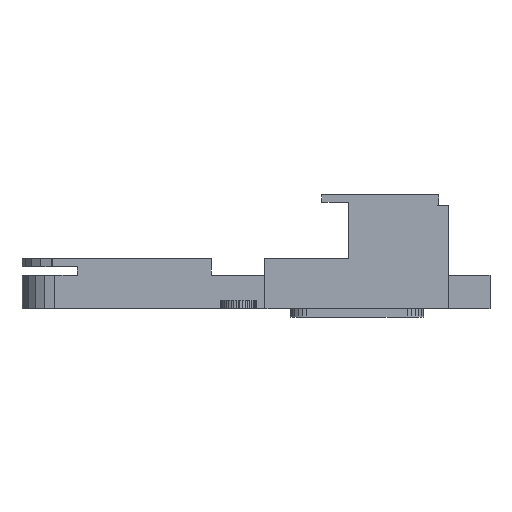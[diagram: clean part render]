
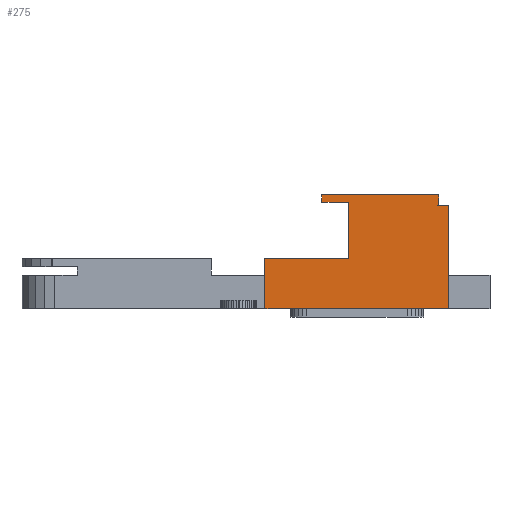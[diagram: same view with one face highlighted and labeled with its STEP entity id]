
A CAD part, front view. The second image highlights one B-rep face of the part: STEP entity #275.
In plain terms, the highlighted planar face has unit normal (0, -1, 0).
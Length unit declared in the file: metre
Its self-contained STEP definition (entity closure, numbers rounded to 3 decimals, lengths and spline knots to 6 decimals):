
#275=ADVANCED_FACE('0:2175',(#930),#931,.T.);
#930=FACE_OUTER_BOUND('',#1837,.T.);
#931=PLANE('',#1838);
#1837=EDGE_LOOP('',(#4191,#4192,#4193,#4194,#4195,#4196,#4197,#4198,#4199,#4200));
#1838=AXIS2_PLACEMENT_3D('',#4201,#4202,#4203);
#4191=ORIENTED_EDGE('',*,*,#6850,.F.);
#4192=ORIENTED_EDGE('',*,*,#6811,.F.);
#4193=ORIENTED_EDGE('',*,*,#6958,.T.);
#4194=ORIENTED_EDGE('',*,*,#6971,.T.);
#4195=ORIENTED_EDGE('',*,*,#6972,.F.);
#4196=ORIENTED_EDGE('',*,*,#6973,.T.);
#4197=ORIENTED_EDGE('',*,*,#6974,.T.);
#4198=ORIENTED_EDGE('',*,*,#6975,.T.);
#4199=ORIENTED_EDGE('',*,*,#6976,.T.);
#4200=ORIENTED_EDGE('',*,*,#6977,.F.);
#4201=CARTESIAN_POINT('',(0.019235,0.127931,0.01905));
#4202=DIRECTION('',(0.0,-1.,0.));
#4203=DIRECTION('',(0.0,0.,-1.));
#6811=EDGE_CURVE('0:2646',#8501,#8503,#8504,.T.);
#6850=EDGE_CURVE('0:2763',#8503,#8570,#8571,.T.);
#6958=EDGE_CURVE('0:3087',#8501,#8783,#8785,.T.);
#6971=EDGE_CURVE('0:3126',#8783,#8810,#8811,.T.);
#6972=EDGE_CURVE('0:3129',#8812,#8810,#8813,.T.);
#6973=EDGE_CURVE('0:3132',#8812,#8814,#8815,.T.);
#6974=EDGE_CURVE('0:3135',#8814,#8816,#8817,.T.);
#6975=EDGE_CURVE('0:3138',#8816,#8818,#8819,.T.);
#6976=EDGE_CURVE('0:3141',#8818,#8820,#8821,.T.);
#6977=EDGE_CURVE('0:3144',#8570,#8820,#8822,.T.);
#8501=VERTEX_POINT('',#11246);
#8503=VERTEX_POINT('',#11249);
#8504=LINE('',#11250,#11251);
#8570=VERTEX_POINT('',#11355);
#8571=LINE('',#11356,#11357);
#8783=VERTEX_POINT('',#11675);
#8785=LINE('',#11678,#11679);
#8810=VERTEX_POINT('',#11716);
#8811=LINE('',#11717,#11718);
#8812=VERTEX_POINT('',#11719);
#8813=LINE('',#11720,#11721);
#8814=VERTEX_POINT('',#11722);
#8815=LINE('',#11723,#11724);
#8816=VERTEX_POINT('',#11725);
#8817=LINE('',#11726,#11727);
#8818=VERTEX_POINT('',#11728);
#8819=LINE('',#11729,#11730);
#8820=VERTEX_POINT('',#11731);
#8821=LINE('',#11732,#11733);
#8822=LINE('',#11734,#11735);
#11246=CARTESIAN_POINT('',(0.012091,0.127931,0.));
#11249=CARTESIAN_POINT('',(0.012091,0.127931,0.01905));
#11250=CARTESIAN_POINT('',(0.012091,0.127931,0.));
#11251=VECTOR('',#13805,1.0);
#11355=CARTESIAN_POINT('',(0.043841,0.127931,0.01905));
#11356=CARTESIAN_POINT('',(0.012091,0.127931,0.01905));
#11357=VECTOR('',#13844,1.0);
#11675=CARTESIAN_POINT('',(0.081941,0.127931,0.));
#11678=CARTESIAN_POINT('',(0.012091,0.127931,0.));
#11679=VECTOR('',#13952,1.0);
#11716=CARTESIAN_POINT('',(0.081941,0.127931,0.03937));
#11717=CARTESIAN_POINT('',(0.081941,0.127931,0.));
#11718=VECTOR('',#13965,1.0);
#11719=CARTESIAN_POINT('',(0.078131,0.127931,0.03937));
#11720=CARTESIAN_POINT('',(0.078131,0.127931,0.03937));
#11721=VECTOR('',#13966,1.0);
#11722=CARTESIAN_POINT('',(0.078131,0.127931,0.04318));
#11723=CARTESIAN_POINT('',(0.078131,0.127931,0.03937));
#11724=VECTOR('',#13967,1.0);
#11725=CARTESIAN_POINT('',(0.033681,0.127931,0.04318));
#11726=CARTESIAN_POINT('',(0.078131,0.127931,0.04318));
#11727=VECTOR('',#13968,1.0);
#11728=CARTESIAN_POINT('',(0.033681,0.127931,0.040513));
#11729=CARTESIAN_POINT('',(0.033681,0.127931,0.04318));
#11730=VECTOR('',#13969,1.0);
#11731=CARTESIAN_POINT('',(0.043841,0.127931,0.040513));
#11732=CARTESIAN_POINT('',(0.033681,0.127931,0.040513));
#11733=VECTOR('',#13970,1.0);
#11734=CARTESIAN_POINT('',(0.043841,0.127931,0.01905));
#11735=VECTOR('',#13971,1.0);
#13805=DIRECTION('',(0.0,0.,1.));
#13844=DIRECTION('',(1.0,0.0,0.0));
#13952=DIRECTION('',(1.0,0.0,0.0));
#13965=DIRECTION('',(0.0,0.,1.));
#13966=DIRECTION('',(1.0,0.0,0.0));
#13967=DIRECTION('',(0.0,0.0,1.0));
#13968=DIRECTION('',(-1.0,0.0,0.0));
#13969=DIRECTION('',(0.0,0.0,-1.0));
#13970=DIRECTION('',(1.0,0.0,0.0));
#13971=DIRECTION('',(0.0,0.0,1.0));
